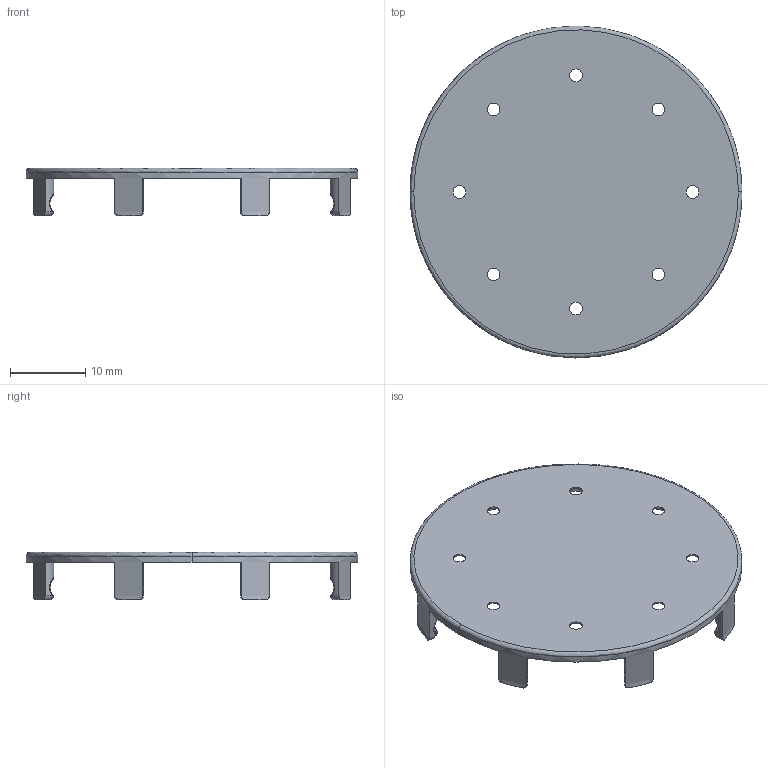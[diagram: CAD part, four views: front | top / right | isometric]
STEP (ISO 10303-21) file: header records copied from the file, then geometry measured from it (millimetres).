
FILE_DESCRIPTION (( 'STEP AP214' ), '1' );
FILE_NAME ('Imura_V3_Cylinder_Cap.step', '2015-04-30T21:14:59', ( 'WarFairy' ), ( '' ), 'SwSTEP 2.0', 'SolidWorks 2013', '' );
FILE_SCHEMA (( 'AUTOMOTIVE_DESIGN' ));
Length unit declared in the file: millimetre
Products named in the file (1): Imura_V3_Cylinder_Cap
Bounding box: 44 x 44 x 6.3 mm (x, y, z)
Volume: 1782.3 mm3; surface area: 3767.8 mm2
Topology: 1 solids, 1 shells, 102 faces, 258 edges, 166 vertices
Faces by surface type: cylinder 46, bspline 38, plane 18
Entity records: 9437 total; most frequent: CARTESIAN_POINT 7095, ORIENTED_EDGE 516, DIRECTION 446, EDGE_CURVE 258, AXIS2_PLACEMENT_3D 196, VERTEX_POINT 166, CIRCLE 131, EDGE_LOOP 126
